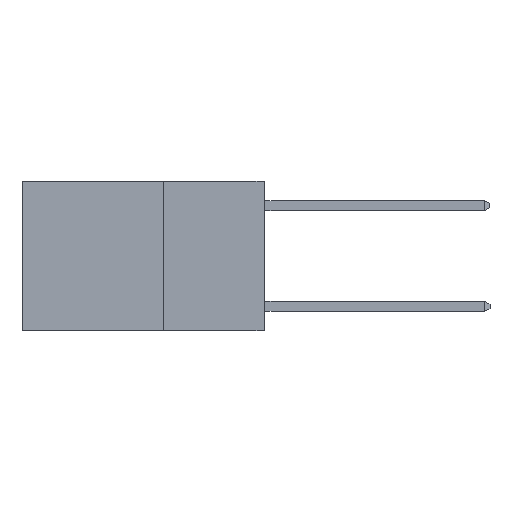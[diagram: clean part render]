
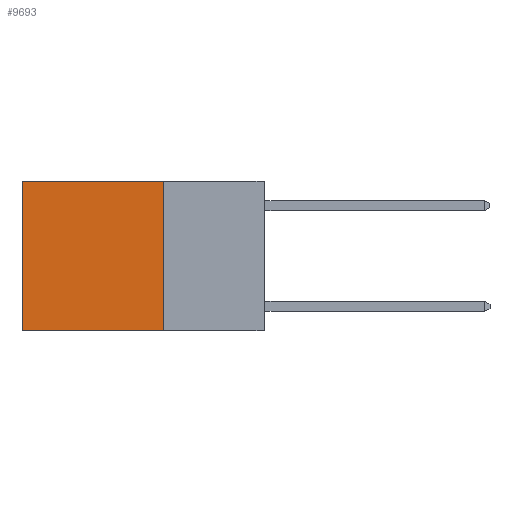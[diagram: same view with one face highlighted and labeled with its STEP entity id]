
A CAD part, left-side view. The second image highlights one B-rep face of the part: STEP entity #9693.
In plain terms, the highlighted planar face has unit normal (-1, 0, 0).
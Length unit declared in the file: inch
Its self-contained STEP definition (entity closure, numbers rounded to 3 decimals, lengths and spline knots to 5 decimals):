
#33 = ORIENTED_EDGE ( 'NONE', *, *, #4067, .F. ) ;
#733 = ORIENTED_EDGE ( 'NONE', *, *, #2471, .T. ) ;
#760 = LINE ( 'NONE', #2791, #4922 ) ;
#761 = VECTOR ( 'NONE', #5234, 39.37008 ) ;
#973 = DIRECTION ( 'NONE',  ( 1., 0., 0. ) ) ;
#1300 = CARTESIAN_POINT ( 'NONE',  ( 0.2625, 0.25, -0.37 ) ) ;
#1605 = FACE_OUTER_BOUND ( 'NONE', #6472, .T. ) ;
#1777 = EDGE_CURVE ( 'NONE', #4584, #3184, #7454, .T. ) ;
#2143 = ORIENTED_EDGE ( 'NONE', *, *, #5819, .F. ) ;
#2471 = EDGE_CURVE ( 'NONE', #5582, #4584, #7041, .T. ) ;
#2544 = CARTESIAN_POINT ( 'NONE',  ( 0.2625, 0.25, 0. ) ) ;
#2791 = CARTESIAN_POINT ( 'NONE',  ( 0.2625, 0.25, 0. ) ) ;
#2849 = LINE ( 'NONE', #1300, #4493 ) ;
#3178 = CARTESIAN_POINT ( 'NONE',  ( 0.2625, 0.25, 0. ) ) ;
#3184 = VERTEX_POINT ( 'NONE', #7425 ) ;
#3725 = CARTESIAN_POINT ( 'NONE',  ( 0.2625, 0.25, -0.37 ) ) ;
#4067 = EDGE_CURVE ( 'NONE', #4619, #3184, #2849, .T. ) ;
#4493 = VECTOR ( 'NONE', #6222, 39.37008 ) ;
#4584 = VERTEX_POINT ( 'NONE', #6085 ) ;
#4619 = VERTEX_POINT ( 'NONE', #3725 ) ;
#4922 = VECTOR ( 'NONE', #7626, 39.37008 ) ;
#5234 = DIRECTION ( 'NONE',  ( 0., 1., 0. ) ) ;
#5315 = VECTOR ( 'NONE', #10109, 39.37008 ) ;
#5582 = VERTEX_POINT ( 'NONE', #2544 ) ;
#5819 = EDGE_CURVE ( 'NONE', #5582, #4619, #760, .T. ) ;
#5913 = CARTESIAN_POINT ( 'NONE',  ( 0.2625, 0.25, 0. ) ) ;
#6085 = CARTESIAN_POINT ( 'NONE',  ( 0.2625, 0.6, 0. ) ) ;
#6222 = DIRECTION ( 'NONE',  ( 0., 1., 0. ) ) ;
#6472 = EDGE_LOOP ( 'NONE', ( #9020, #33, #2143, #733 ) ) ;
#6668 = PLANE ( 'NONE',  #7678 ) ;
#6699 = DIRECTION ( 'NONE',  ( 0., 0., -1. ) ) ;
#7041 = LINE ( 'NONE', #3178, #761 ) ;
#7425 = CARTESIAN_POINT ( 'NONE',  ( 0.2625, 0.6, -0.37 ) ) ;
#7454 = LINE ( 'NONE', #10068, #5315 ) ;
#7626 = DIRECTION ( 'NONE',  ( 0., 0., -1. ) ) ;
#7678 = AXIS2_PLACEMENT_3D ( 'NONE', #5913, #973, #6699 ) ;
#9020 = ORIENTED_EDGE ( 'NONE', *, *, #1777, .T. ) ;
#9693 = ADVANCED_FACE ( 'NONE', ( #1605 ), #6668, .F. ) ;
#10068 = CARTESIAN_POINT ( 'NONE',  ( 0.2625, 0.6, 0. ) ) ;
#10109 = DIRECTION ( 'NONE',  ( 0., 0., -1. ) ) ;
